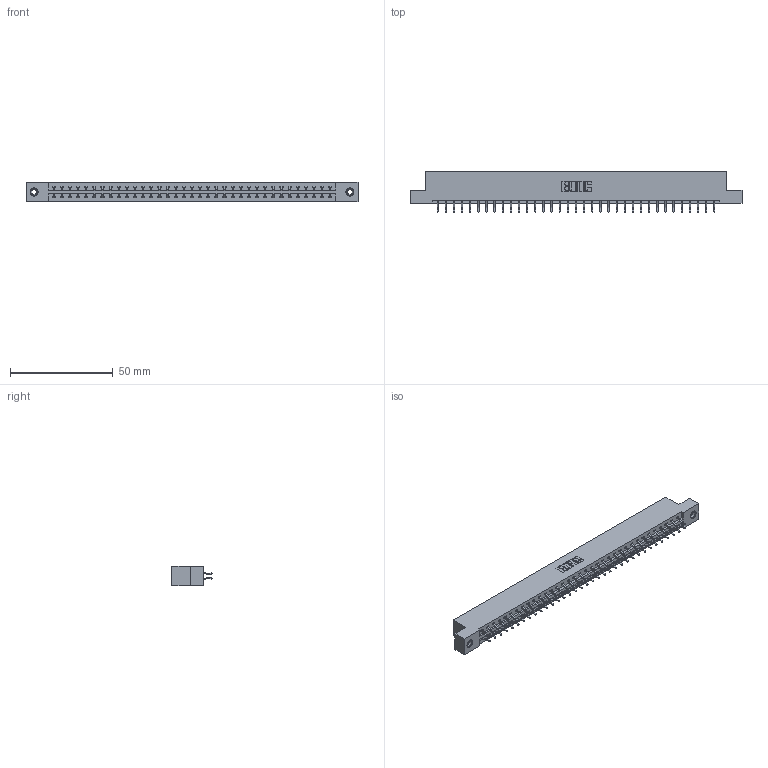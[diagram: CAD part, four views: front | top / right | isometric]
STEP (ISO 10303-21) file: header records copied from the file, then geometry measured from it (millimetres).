
FILE_DESCRIPTION (( 'STEP AP203' ), '1' );
FILE_NAME ('387-070-556-208.STEP', '2018-09-22T17:16:06', ( '' ), ( '' ), 'SwSTEP 2.0', 'SolidWorks 2016', '' );
FILE_SCHEMA (( 'CONFIG_CONTROL_DESIGN' ));
Length unit declared in the file: inch
Products named in the file (4): 337 Part_Flush Mounting Lugs - 0.156 Dia-TI; 345-292-001_556 Tail; 345-250-001_345-250-003-102; 387-070-556-208
Assembly tree (73 placements, depth 2):
  387-070-556-208
    337 Part_Flush Mounting Lugs - 0.156 Dia-TI
    345-292-001_556 Tail  x70
    345-250-001_345-250-003-102  x2
Bounding box: 161.7 x 19.57 x 9.4 mm (x, y, z)
Volume: 16938.4 mm3; surface area: 19030.9 mm2
Topology: 73 solids, 73 shells, 4374 faces, 12977 edges, 8550 vertices
Faces by surface type: plane 3042, cylinder 1316, cone 12, torus 4
Entity records: 29448 total; most frequent: CARTESIAN_POINT 4961, ORIENTED_EDGE 4878, DIRECTION 4253, EDGE_CURVE 2439, LINE 2283, VECTOR 2283, VERTEX_POINT 1620, AXIS2_PLACEMENT_3D 985
